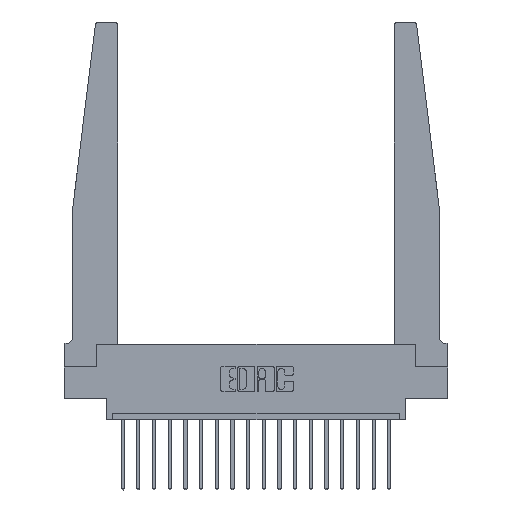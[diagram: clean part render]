
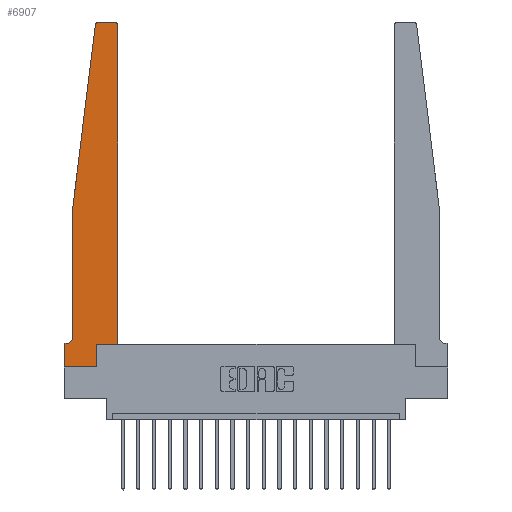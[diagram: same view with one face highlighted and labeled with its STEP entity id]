
A CAD part, top view. The second image highlights one B-rep face of the part: STEP entity #6907.
In plain terms, the highlighted planar face has unit normal (0, 0, 1).
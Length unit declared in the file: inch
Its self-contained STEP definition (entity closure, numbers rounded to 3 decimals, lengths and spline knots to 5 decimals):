
#416 = ORIENTED_EDGE ( 'NONE', *, *, #8743, .T. ) ;
#524 = ORIENTED_EDGE ( 'NONE', *, *, #17169, .T. ) ;
#1089 = VERTEX_POINT ( 'NONE', #19182 ) ;
#1152 = VERTEX_POINT ( 'NONE', #2968 ) ;
#1696 = CARTESIAN_POINT ( 'NONE',  ( 0.065, 1.25, 0.37 ) ) ;
#2026 = VECTOR ( 'NONE', #17059, 39.37008 ) ;
#2459 = LINE ( 'NONE', #2467, #13908 ) ;
#2467 = CARTESIAN_POINT ( 'NONE',  ( 0., 0., 0.37 ) ) ;
#2759 = VECTOR ( 'NONE', #10606, 39.37008 ) ;
#2902 = CARTESIAN_POINT ( 'NONE',  ( 0., 0.1875, 0.37 ) ) ;
#2948 = DIRECTION ( 'NONE',  ( 0., 0., 1. ) ) ;
#2968 = CARTESIAN_POINT ( 'NONE',  ( 0.395, 2.75, 0.37 ) ) ;
#3079 = LINE ( 'NONE', #14955, #17981 ) ;
#3086 = CARTESIAN_POINT ( 'NONE',  ( 0.27653, 2.72, 0.37 ) ) ;
#3250 = VECTOR ( 'NONE', #15961, 39.37008 ) ;
#3402 = DIRECTION ( 'NONE',  ( 1., 0., 0. ) ) ;
#3600 = VERTEX_POINT ( 'NONE', #6012 ) ;
#3818 = EDGE_CURVE ( 'NONE', #13366, #7627, #17352, .T. ) ;
#3864 = DIRECTION ( 'NONE',  ( 0., 1., 0. ) ) ;
#3865 = AXIS2_PLACEMENT_3D ( 'NONE', #3086, #16615, #16484 ) ;
#3994 = EDGE_CURVE ( 'NONE', #7627, #9470, #2459, .T. ) ;
#4224 = VERTEX_POINT ( 'NONE', #1696 ) ;
#4307 = CARTESIAN_POINT ( 'NONE',  ( 0.425, 0.18, 0.37 ) ) ;
#4515 = ORIENTED_EDGE ( 'NONE', *, *, #17622, .T. ) ;
#4589 = LINE ( 'NONE', #10635, #13976 ) ;
#4681 = CARTESIAN_POINT ( 'NONE',  ( 0.395, 2.72, 0.37 ) ) ;
#4714 = CARTESIAN_POINT ( 'NONE',  ( 0.2605, 0.18, 0.37 ) ) ;
#4764 = ORIENTED_EDGE ( 'NONE', *, *, #12190, .T. ) ;
#5078 = VERTEX_POINT ( 'NONE', #4714 ) ;
#5467 = EDGE_LOOP ( 'NONE', ( #14516, #524, #16855, #416, #4764, #5563, #8793, #4515, #12589, #12570, #7376, #6921 ) ) ;
#5563 = ORIENTED_EDGE ( 'NONE', *, *, #3818, .T. ) ;
#5976 = DIRECTION ( 'NONE',  ( -1., 0., 0. ) ) ;
#6012 = CARTESIAN_POINT ( 'NONE',  ( 0.27653, 2.75, 0.37 ) ) ;
#6027 = DIRECTION ( 'NONE',  ( 0., 1., 0. ) ) ;
#6205 = EDGE_CURVE ( 'NONE', #16009, #5078, #10768, .T. ) ;
#6530 = CARTESIAN_POINT ( 'NONE',  ( 0.065, 0.1875, 0.37 ) ) ;
#6907 = ADVANCED_FACE ( 'NONE', ( #19141 ), #12883, .T. ) ;
#6921 = ORIENTED_EDGE ( 'NONE', *, *, #8398, .T. ) ;
#7160 = EDGE_CURVE ( 'NONE', #10425, #1089, #3079, .T. ) ;
#7189 = CIRCLE ( 'NONE', #7451, 0.03 ) ;
#7265 = VERTEX_POINT ( 'NONE', #9450 ) ;
#7376 = ORIENTED_EDGE ( 'NONE', *, *, #7160, .T. ) ;
#7451 = AXIS2_PLACEMENT_3D ( 'NONE', #4681, #2948, #3402 ) ;
#7627 = VERTEX_POINT ( 'NONE', #2902 ) ;
#7942 = VECTOR ( 'NONE', #3864, 39.37008 ) ;
#8279 = LINE ( 'NONE', #9744, #2026 ) ;
#8398 = EDGE_CURVE ( 'NONE', #1089, #1152, #7189, .T. ) ;
#8509 = DIRECTION ( 'NONE',  ( 1., 0., 0. ) ) ;
#8535 = DIRECTION ( 'NONE',  ( 0., 0., 1. ) ) ;
#8743 = EDGE_CURVE ( 'NONE', #4224, #7265, #19086, .T. ) ;
#8793 = ORIENTED_EDGE ( 'NONE', *, *, #3994, .T. ) ;
#8945 = DIRECTION ( 'NONE',  ( 0., 0., -1. ) ) ;
#9180 = DIRECTION ( 'NONE',  ( 1., 0., 0. ) ) ;
#9450 = CARTESIAN_POINT ( 'NONE',  ( 0.065, 0.2375, 0.37 ) ) ;
#9470 = VERTEX_POINT ( 'NONE', #11695 ) ;
#9516 = VERTEX_POINT ( 'NONE', #10151 ) ;
#9744 = CARTESIAN_POINT ( 'NONE',  ( 0.25, 2.75, 0.37 ) ) ;
#9901 = CARTESIAN_POINT ( 'NONE',  ( 0.065, 1.25, 0.37 ) ) ;
#9957 = CARTESIAN_POINT ( 'NONE',  ( 0.2605, 0., 0.37 ) ) ;
#10077 = DIRECTION ( 'NONE',  ( 1., 0., 0. ) ) ;
#10151 = CARTESIAN_POINT ( 'NONE',  ( 0.24675, 2.72367, 0.37 ) ) ;
#10425 = VERTEX_POINT ( 'NONE', #4307 ) ;
#10606 = DIRECTION ( 'NONE',  ( -0.122, -0.992, 0. ) ) ;
#10635 = CARTESIAN_POINT ( 'NONE',  ( 0., 0., 0.37 ) ) ;
#10641 = LINE ( 'NONE', #19052, #12742 ) ;
#10768 = LINE ( 'NONE', #17200, #7942 ) ;
#11695 = CARTESIAN_POINT ( 'NONE',  ( 0., 0., 0.37 ) ) ;
#12174 = EDGE_CURVE ( 'NONE', #9516, #4224, #13249, .T. ) ;
#12190 = EDGE_CURVE ( 'NONE', #7265, #13366, #16044, .T. ) ;
#12570 = ORIENTED_EDGE ( 'NONE', *, *, #14000, .T. ) ;
#12589 = ORIENTED_EDGE ( 'NONE', *, *, #6205, .T. ) ;
#12742 = VECTOR ( 'NONE', #8509, 39.37008 ) ;
#12883 = PLANE ( 'NONE',  #14496 ) ;
#12891 = DIRECTION ( 'NONE',  ( 0., -1., 0. ) ) ;
#13249 = LINE ( 'NONE', #18032, #2759 ) ;
#13366 = VERTEX_POINT ( 'NONE', #18693 ) ;
#13908 = VECTOR ( 'NONE', #12891, 39.37008 ) ;
#13976 = VECTOR ( 'NONE', #9180, 39.37008 ) ;
#14000 = EDGE_CURVE ( 'NONE', #5078, #10425, #10641, .T. ) ;
#14496 = AXIS2_PLACEMENT_3D ( 'NONE', #17491, #8535, #10077 ) ;
#14516 = ORIENTED_EDGE ( 'NONE', *, *, #17492, .T. ) ;
#14626 = CIRCLE ( 'NONE', #3865, 0.03 ) ;
#14955 = CARTESIAN_POINT ( 'NONE',  ( 0.425, 0.18, 0.37 ) ) ;
#15325 = DIRECTION ( 'NONE',  ( -1., 0., 0. ) ) ;
#15423 = AXIS2_PLACEMENT_3D ( 'NONE', #17910, #8945, #5976 ) ;
#15961 = DIRECTION ( 'NONE',  ( 0., -1., 0. ) ) ;
#16009 = VERTEX_POINT ( 'NONE', #9957 ) ;
#16044 = CIRCLE ( 'NONE', #15423, 0.05 ) ;
#16484 = DIRECTION ( 'NONE',  ( 1., 0., 0. ) ) ;
#16615 = DIRECTION ( 'NONE',  ( 0., 0., 1. ) ) ;
#16855 = ORIENTED_EDGE ( 'NONE', *, *, #12174, .T. ) ;
#17059 = DIRECTION ( 'NONE',  ( -1., 0., 0. ) ) ;
#17169 = EDGE_CURVE ( 'NONE', #3600, #9516, #14626, .T. ) ;
#17200 = CARTESIAN_POINT ( 'NONE',  ( 0.2605, 0.18, 0.37 ) ) ;
#17352 = LINE ( 'NONE', #6530, #18794 ) ;
#17492 = EDGE_CURVE ( 'NONE', #1152, #3600, #8279, .T. ) ;
#17491 = CARTESIAN_POINT ( 'NONE',  ( 0., 0.1875, 0.37 ) ) ;
#17622 = EDGE_CURVE ( 'NONE', #9470, #16009, #4589, .T. ) ;
#17910 = CARTESIAN_POINT ( 'NONE',  ( 0.015, 0.2375, 0.37 ) ) ;
#17981 = VECTOR ( 'NONE', #6027, 39.37008 ) ;
#18032 = CARTESIAN_POINT ( 'NONE',  ( 0.065, 1.25, 0.37 ) ) ;
#18693 = CARTESIAN_POINT ( 'NONE',  ( 0.015, 0.1875, 0.37 ) ) ;
#18794 = VECTOR ( 'NONE', #15325, 39.37008 ) ;
#19052 = CARTESIAN_POINT ( 'NONE',  ( 0.425, 0.18, 0.37 ) ) ;
#19086 = LINE ( 'NONE', #9901, #3250 ) ;
#19141 = FACE_OUTER_BOUND ( 'NONE', #5467, .T. ) ;
#19182 = CARTESIAN_POINT ( 'NONE',  ( 0.425, 2.72, 0.37 ) ) ;
